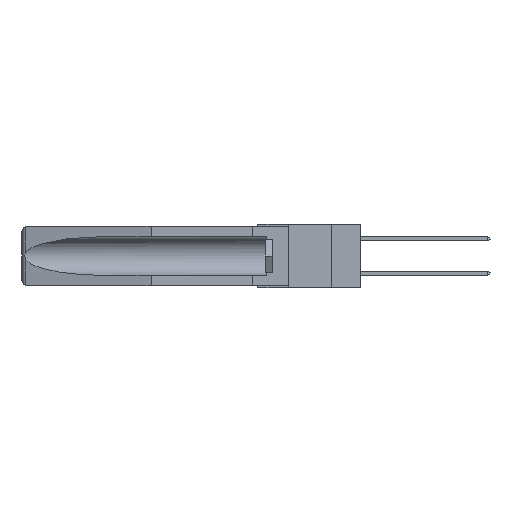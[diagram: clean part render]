
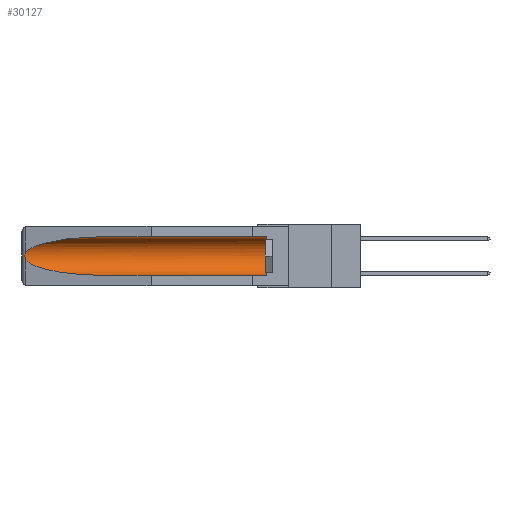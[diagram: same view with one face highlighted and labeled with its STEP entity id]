
A CAD part, left-side view. The second image highlights one B-rep face of the part: STEP entity #30127.
In plain terms, the highlighted cylindrical face has radius 2.857 mm (diameter 5.715 mm), a partial arc.
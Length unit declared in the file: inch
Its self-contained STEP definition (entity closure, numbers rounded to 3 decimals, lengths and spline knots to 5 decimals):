
#163 = ORIENTED_EDGE ( 'NONE', *, *, #25531, .T. ) ;
#365 = CARTESIAN_POINT ( 'NONE',  ( 0.155, 0.126, -0.1715 ) ) ;
#400 = CARTESIAN_POINT ( 'NONE',  ( 0.155, 1.07973, -0.059 ) ) ;
#1125 = DIRECTION ( 'NONE',  ( 0., 0., 1. ) ) ;
#1235 = DIRECTION ( 'NONE',  ( 0., 1., 0. ) ) ;
#1613 = VERTEX_POINT ( 'NONE', #400 ) ;
#1976 = CARTESIAN_POINT ( 'NONE',  ( 0.25451, 1.48313, -0.09465 ) ) ;
#2303 = AXIS2_PLACEMENT_3D ( 'NONE', #365, #8649, #1125 ) ;
#2414 = FACE_OUTER_BOUND ( 'NONE', #23494, .T. ) ;
#2515 = CARTESIAN_POINT ( 'NONE',  ( 0.26655, 1.53094, -0.18657 ) ) ;
#2833 = VERTEX_POINT ( 'NONE', #3811 ) ;
#3811 = CARTESIAN_POINT ( 'NONE',  ( 0.155, 1.07973, -0.284 ) ) ;
#4990 = CARTESIAN_POINT ( 'NONE',  ( 0.26537, 1.52718, -0.19328 ) ) ;
#6110 = EDGE_CURVE ( 'NONE', #14182, #1613, #9347, .T. ) ;
#6719 =( BOUNDED_CURVE ( )  B_SPLINE_CURVE ( 3, ( #19159, #19266, #1976, #9157 ),
 .UNSPECIFIED., .F., .F. ) 
 B_SPLINE_CURVE_WITH_KNOTS ( ( 4, 4 ),
 ( 4.71239, 6.08839 ),
 .UNSPECIFIED. ) 
 CURVE ( )  GEOMETRIC_REPRESENTATION_ITEM ( )  RATIONAL_B_SPLINE_CURVE ( ( 1., 0.848, 0.848, 1. ) ) 
 REPRESENTATION_ITEM ( '' )  );
#7077 = ORIENTED_EDGE ( 'NONE', *, *, #6110, .T. ) ;
#7263 = CARTESIAN_POINT ( 'NONE',  ( 0.155, -0.30754, -0.284 ) ) ;
#7273 = CARTESIAN_POINT ( 'NONE',  ( 0.2675, 1.53308, -0.17534 ) ) ;
#7932 = CARTESIAN_POINT ( 'NONE',  ( 0.26537, 1.52718, -0.19328 ) ) ;
#8624 = EDGE_CURVE ( 'NONE', #21053, #14182, #31396, .T. ) ;
#8649 = DIRECTION ( 'NONE',  ( 0., -1., 0. ) ) ;
#9157 = CARTESIAN_POINT ( 'NONE',  ( 0.26537, 1.52718, -0.14972 ) ) ;
#9310 = CARTESIAN_POINT ( 'NONE',  ( 0.21114, 1.30732, -0.284 ) ) ;
#9347 = LINE ( 'NONE', #21390, #21951 ) ;
#9532 = AXIS2_PLACEMENT_3D ( 'NONE', #29811, #32300, #19387 ) ;
#9714 = ORIENTED_EDGE ( 'NONE', *, *, #30796, .T. ) ;
#9988 = CARTESIAN_POINT ( 'NONE',  ( 0.26537, 1.52718, -0.14972 ) ) ;
#11596 = EDGE_CURVE ( 'NONE', #21053, #2833, #30001, .T. ) ;
#11615 = CARTESIAN_POINT ( 'NONE',  ( 0.26537, 1.52718, -0.14972 ) ) ;
#12327 = CARTESIAN_POINT ( 'NONE',  ( 0.2673, 1.5327, -0.16383 ) ) ;
#13465 = EDGE_CURVE ( 'NONE', #19683, #21931, #16830, .T. ) ;
#14182 = VERTEX_POINT ( 'NONE', #24047 ) ;
#16830 = B_SPLINE_CURVE_WITH_KNOTS ( 'NONE', 3,
 ( #9988, #17491, #27319, #12327, #17274, #7273, #19795, #2515, #20121, #4990 ),
 .UNSPECIFIED., .F., .F.,
 ( 4, 2, 2, 2, 4 ),
 ( 0., 0.00029, 0.00058, 0.00087, 0.00117 ),
 .UNSPECIFIED. ) ;
#17274 = CARTESIAN_POINT ( 'NONE',  ( 0.2675, 1.53308, -0.16763 ) ) ;
#17491 = CARTESIAN_POINT ( 'NONE',  ( 0.26597, 1.52961, -0.15275 ) ) ;
#17538 = ORIENTED_EDGE ( 'NONE', *, *, #13465, .T. ) ;
#18997 = CARTESIAN_POINT ( 'NONE',  ( 0.26537, 1.52718, -0.19328 ) ) ;
#19139 = CARTESIAN_POINT ( 'NONE',  ( 0.155, 0.126, -0.284 ) ) ;
#19159 = CARTESIAN_POINT ( 'NONE',  ( 0.155, 1.07973, -0.059 ) ) ;
#19266 = CARTESIAN_POINT ( 'NONE',  ( 0.21114, 1.30732, -0.059 ) ) ;
#19387 = DIRECTION ( 'NONE',  ( 0., 0., 1. ) ) ;
#19683 = VERTEX_POINT ( 'NONE', #11615 ) ;
#19795 = CARTESIAN_POINT ( 'NONE',  ( 0.2673, 1.53269, -0.17917 ) ) ;
#20010 = CYLINDRICAL_SURFACE ( 'NONE', #9532, 0.1125 ) ;
#20121 = CARTESIAN_POINT ( 'NONE',  ( 0.26597, 1.5296, -0.19026 ) ) ;
#21053 = VERTEX_POINT ( 'NONE', #19139 ) ;
#21390 = CARTESIAN_POINT ( 'NONE',  ( 0.155, -0.30754, -0.059 ) ) ;
#21931 = VERTEX_POINT ( 'NONE', #7932 ) ;
#21951 = VECTOR ( 'NONE', #1235, 39.37008 ) ;
#23494 = EDGE_LOOP ( 'NONE', ( #163, #17538, #9714, #26557, #25971, #7077 ) ) ;
#24047 = CARTESIAN_POINT ( 'NONE',  ( 0.155, 0.126, -0.059 ) ) ;
#24743 = DIRECTION ( 'NONE',  ( 0., 1., 0. ) ) ;
#25531 = EDGE_CURVE ( 'NONE', #1613, #19683, #6719, .T. ) ;
#25971 = ORIENTED_EDGE ( 'NONE', *, *, #8624, .T. ) ;
#26557 = ORIENTED_EDGE ( 'NONE', *, *, #11596, .F. ) ;
#27319 = CARTESIAN_POINT ( 'NONE',  ( 0.26654, 1.53092, -0.15636 ) ) ;
#27689 = VECTOR ( 'NONE', #24743, 39.37008 ) ;
#27701 =( BOUNDED_CURVE ( )  B_SPLINE_CURVE ( 3, ( #18997, #28694, #9310, #29232 ),
 .UNSPECIFIED., .F., .F. ) 
 B_SPLINE_CURVE_WITH_KNOTS ( ( 4, 4 ),
 ( 0.1948, 1.5708 ),
 .UNSPECIFIED. ) 
 CURVE ( )  GEOMETRIC_REPRESENTATION_ITEM ( )  RATIONAL_B_SPLINE_CURVE ( ( 1., 0.848, 0.848, 1. ) ) 
 REPRESENTATION_ITEM ( '' )  );
#28694 = CARTESIAN_POINT ( 'NONE',  ( 0.25451, 1.48313, -0.24835 ) ) ;
#29232 = CARTESIAN_POINT ( 'NONE',  ( 0.155, 1.07973, -0.284 ) ) ;
#29811 = CARTESIAN_POINT ( 'NONE',  ( 0.155, -0.30754, -0.1715 ) ) ;
#30001 = LINE ( 'NONE', #7263, #27689 ) ;
#30127 = ADVANCED_FACE ( 'NONE', ( #2414 ), #20010, .F. ) ;
#30796 = EDGE_CURVE ( 'NONE', #21931, #2833, #27701, .T. ) ;
#31396 = CIRCLE ( 'NONE', #2303, 0.1125 ) ;
#32300 = DIRECTION ( 'NONE',  ( 0., 1., 0. ) ) ;
